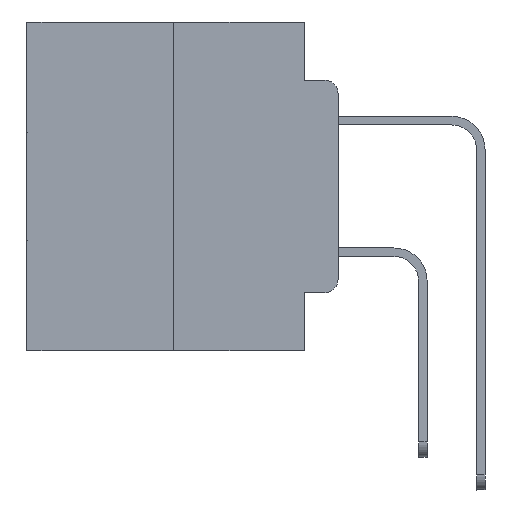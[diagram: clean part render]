
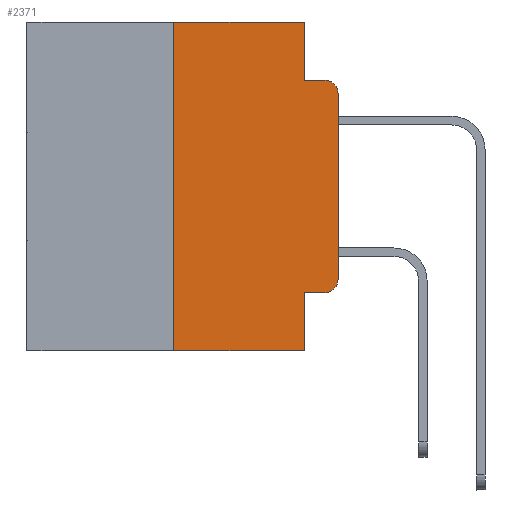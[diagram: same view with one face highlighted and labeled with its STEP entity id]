
A CAD part, left-side view. The second image highlights one B-rep face of the part: STEP entity #2371.
In plain terms, the highlighted planar face has unit normal (-1, 0, 0).
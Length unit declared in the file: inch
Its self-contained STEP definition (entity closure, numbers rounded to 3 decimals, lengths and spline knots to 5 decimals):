
#307 = CIRCLE ( 'NONE', #26143, 0.02 ) ;
#537 = AXIS2_PLACEMENT_3D ( 'NONE', #16613, #3156, #18824 ) ;
#1078 = VECTOR ( 'NONE', #20086, 39.37008 ) ;
#1168 = LINE ( 'NONE', #25371, #24194 ) ;
#1303 = ORIENTED_EDGE ( 'NONE', *, *, #1861, .F. ) ;
#1315 = CARTESIAN_POINT ( 'NONE',  ( 0., 0.051, -0.4115 ) ) ;
#1741 = CARTESIAN_POINT ( 'NONE',  ( 0., 0., 0. ) ) ;
#1861 = EDGE_CURVE ( 'NONE', #19723, #5303, #24598, .T. ) ;
#2156 = CARTESIAN_POINT ( 'NONE',  ( 0., 0.02, -0.0885 ) ) ;
#2371 = ADVANCED_FACE ( 'NONE', ( #27634 ), #7307, .F. ) ;
#2533 = CARTESIAN_POINT ( 'NONE',  ( 0., 0., -0.3915 ) ) ;
#2622 = VERTEX_POINT ( 'NONE', #2156 ) ;
#2818 = EDGE_CURVE ( 'NONE', #18690, #19723, #15920, .T. ) ;
#3132 = CARTESIAN_POINT ( 'NONE',  ( 0., 0.02, -0.4115 ) ) ;
#3156 = DIRECTION ( 'NONE',  ( -1., 0., 0. ) ) ;
#4259 = VECTOR ( 'NONE', #15205, 39.37008 ) ;
#4740 = CARTESIAN_POINT ( 'NONE',  ( 0., 0.473, 0. ) ) ;
#4825 = DIRECTION ( 'NONE',  ( 0., 0., -1. ) ) ;
#4830 = ORIENTED_EDGE ( 'NONE', *, *, #11454, .F. ) ;
#5153 = ORIENTED_EDGE ( 'NONE', *, *, #25951, .T. ) ;
#5303 = VERTEX_POINT ( 'NONE', #18265 ) ;
#7108 = CARTESIAN_POINT ( 'NONE',  ( 0., 0.473, 0. ) ) ;
#7307 = PLANE ( 'NONE',  #15237 ) ;
#7726 = CARTESIAN_POINT ( 'NONE',  ( 0., 0.051, 0. ) ) ;
#8021 = ORIENTED_EDGE ( 'NONE', *, *, #14619, .F. ) ;
#8408 = CIRCLE ( 'NONE', #537, 0.02 ) ;
#8922 = LINE ( 'NONE', #7726, #12730 ) ;
#9092 = VERTEX_POINT ( 'NONE', #1315 ) ;
#9936 = DIRECTION ( 'NONE',  ( 0., 0., -1. ) ) ;
#10124 = EDGE_CURVE ( 'NONE', #25054, #2622, #24187, .T. ) ;
#10188 = LINE ( 'NONE', #1741, #4259 ) ;
#10476 = CARTESIAN_POINT ( 'NONE',  ( 0., 0.02, -0.3915 ) ) ;
#10956 = CARTESIAN_POINT ( 'NONE',  ( 0., 0.051, -0.0885 ) ) ;
#11454 = EDGE_CURVE ( 'NONE', #5303, #25054, #11581, .T. ) ;
#11581 = LINE ( 'NONE', #13328, #1078 ) ;
#11750 = EDGE_CURVE ( 'NONE', #27462, #2622, #8408, .T. ) ;
#12057 = DIRECTION ( 'NONE',  ( 0., -1., 0. ) ) ;
#12059 = CARTESIAN_POINT ( 'NONE',  ( 0., 0.473, -0.5 ) ) ;
#12730 = VECTOR ( 'NONE', #9936, 39.37008 ) ;
#12731 = DIRECTION ( 'NONE',  ( 0., 0., -1. ) ) ;
#13328 = CARTESIAN_POINT ( 'NONE',  ( 0., 0.051, 0. ) ) ;
#14100 = CARTESIAN_POINT ( 'NONE',  ( 0., 0.25, 0. ) ) ;
#14619 = EDGE_CURVE ( 'NONE', #9092, #21785, #8922, .T. ) ;
#15205 = DIRECTION ( 'NONE',  ( 0., 0., 1. ) ) ;
#15237 = AXIS2_PLACEMENT_3D ( 'NONE', #7108, #20442, #4825 ) ;
#15920 = LINE ( 'NONE', #14100, #22486 ) ;
#16613 = CARTESIAN_POINT ( 'NONE',  ( 0., 0.02, -0.1085 ) ) ;
#17071 = DIRECTION ( 'NONE',  ( 0., 0., 1. ) ) ;
#18115 = ORIENTED_EDGE ( 'NONE', *, *, #10124, .F. ) ;
#18265 = CARTESIAN_POINT ( 'NONE',  ( 0., 0.051, 0. ) ) ;
#18355 = VECTOR ( 'NONE', #26648, 39.37008 ) ;
#18406 = EDGE_CURVE ( 'NONE', #18690, #21785, #28020, .T. ) ;
#18690 = VERTEX_POINT ( 'NONE', #21710 ) ;
#18824 = DIRECTION ( 'NONE',  ( 0., 0., -1. ) ) ;
#18833 = DIRECTION ( 'NONE',  ( 0., -1., 0. ) ) ;
#19128 = VERTEX_POINT ( 'NONE', #3132 ) ;
#19723 = VERTEX_POINT ( 'NONE', #25207 ) ;
#20086 = DIRECTION ( 'NONE',  ( 0., 0., -1. ) ) ;
#20192 = EDGE_LOOP ( 'NONE', ( #5153, #26997, #18115, #4830, #1303, #28728, #26013, #8021, #20804, #21304 ) ) ;
#20373 = EDGE_CURVE ( 'NONE', #9092, #19128, #1168, .T. ) ;
#20442 = DIRECTION ( 'NONE',  ( 1., 0., 0. ) ) ;
#20570 = DIRECTION ( 'NONE',  ( 0., -1., 0. ) ) ;
#20653 = CARTESIAN_POINT ( 'NONE',  ( 0., 0.051, -0.5 ) ) ;
#20804 = ORIENTED_EDGE ( 'NONE', *, *, #20373, .T. ) ;
#21304 = ORIENTED_EDGE ( 'NONE', *, *, #25870, .T. ) ;
#21710 = CARTESIAN_POINT ( 'NONE',  ( 0., 0.25, -0.5 ) ) ;
#21785 = VERTEX_POINT ( 'NONE', #20653 ) ;
#22486 = VECTOR ( 'NONE', #17071, 39.37008 ) ;
#23233 = VECTOR ( 'NONE', #20570, 39.37008 ) ;
#23349 = CARTESIAN_POINT ( 'NONE',  ( 0., 0., -0.1085 ) ) ;
#24187 = LINE ( 'NONE', #10956, #18355 ) ;
#24194 = VECTOR ( 'NONE', #12057, 39.37008 ) ;
#24598 = LINE ( 'NONE', #4740, #23233 ) ;
#25054 = VERTEX_POINT ( 'NONE', #25397 ) ;
#25207 = CARTESIAN_POINT ( 'NONE',  ( 0., 0.25, 0. ) ) ;
#25371 = CARTESIAN_POINT ( 'NONE',  ( 0., 0.051, -0.4115 ) ) ;
#25397 = CARTESIAN_POINT ( 'NONE',  ( 0., 0.051, -0.0885 ) ) ;
#25870 = EDGE_CURVE ( 'NONE', #19128, #26178, #307, .T. ) ;
#25951 = EDGE_CURVE ( 'NONE', #26178, #27462, #10188, .T. ) ;
#25999 = DIRECTION ( 'NONE',  ( -1., 0., 0. ) ) ;
#26013 = ORIENTED_EDGE ( 'NONE', *, *, #18406, .T. ) ;
#26143 = AXIS2_PLACEMENT_3D ( 'NONE', #10476, #25999, #12731 ) ;
#26178 = VERTEX_POINT ( 'NONE', #2533 ) ;
#26648 = DIRECTION ( 'NONE',  ( 0., -1., 0. ) ) ;
#26997 = ORIENTED_EDGE ( 'NONE', *, *, #11750, .T. ) ;
#27462 = VERTEX_POINT ( 'NONE', #23349 ) ;
#27634 = FACE_OUTER_BOUND ( 'NONE', #20192, .T. ) ;
#28020 = LINE ( 'NONE', #12059, #28700 ) ;
#28700 = VECTOR ( 'NONE', #18833, 39.37008 ) ;
#28728 = ORIENTED_EDGE ( 'NONE', *, *, #2818, .F. ) ;
